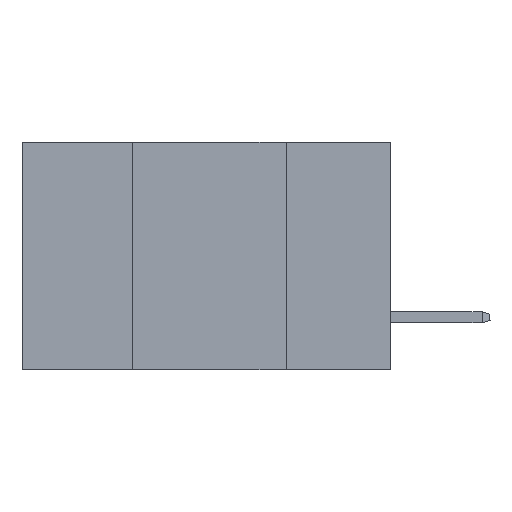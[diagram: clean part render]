
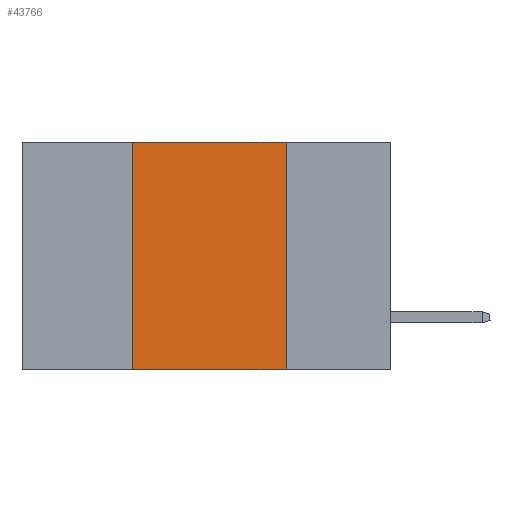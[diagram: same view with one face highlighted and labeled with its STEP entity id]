
A CAD part, left-side view. The second image highlights one B-rep face of the part: STEP entity #43766.
In plain terms, the highlighted planar face has unit normal (-1, 0, 0).
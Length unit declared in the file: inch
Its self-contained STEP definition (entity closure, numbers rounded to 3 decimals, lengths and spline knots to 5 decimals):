
#267 = LINE ( 'NONE', #17194, #22926 ) ;
#1456 = EDGE_CURVE ( 'NONE', #11638, #3674, #27664, .T. ) ;
#1714 = VERTEX_POINT ( 'NONE', #45940 ) ;
#2874 = DIRECTION ( 'NONE',  ( 1., 0., 0. ) ) ;
#2916 = CARTESIAN_POINT ( 'NONE',  ( 0., 0.17, -0.37 ) ) ;
#3674 = VERTEX_POINT ( 'NONE', #2916 ) ;
#4388 = EDGE_CURVE ( 'NONE', #11638, #10976, #28639, .T. ) ;
#6212 = PLANE ( 'NONE',  #17235 ) ;
#9641 = CARTESIAN_POINT ( 'NONE',  ( 0., 0.42, -0.37 ) ) ;
#10976 = VERTEX_POINT ( 'NONE', #39922 ) ;
#11638 = VERTEX_POINT ( 'NONE', #9641 ) ;
#13337 = ORIENTED_EDGE ( 'NONE', *, *, #4388, .F. ) ;
#13346 = EDGE_LOOP ( 'NONE', ( #35513, #32151, #13337, #45210 ) ) ;
#13488 = CARTESIAN_POINT ( 'NONE',  ( 0., 0.17, 0. ) ) ;
#13696 = CARTESIAN_POINT ( 'NONE',  ( 0., 0.42, 0. ) ) ;
#14309 = DIRECTION ( 'NONE',  ( 0., 0., 1. ) ) ;
#16342 = LINE ( 'NONE', #13488, #26004 ) ;
#17088 = CARTESIAN_POINT ( 'NONE',  ( 0., 0.6, 0. ) ) ;
#17194 = CARTESIAN_POINT ( 'NONE',  ( 0., 0.6, 0. ) ) ;
#17235 = AXIS2_PLACEMENT_3D ( 'NONE', #17088, #2874, #39387 ) ;
#17655 = DIRECTION ( 'NONE',  ( 0., -1., 0. ) ) ;
#22926 = VECTOR ( 'NONE', #17655, 39.37008 ) ;
#24451 = DIRECTION ( 'NONE',  ( 0., 0., -1. ) ) ;
#25090 = CARTESIAN_POINT ( 'NONE',  ( 0., 0.6, -0.37 ) ) ;
#26004 = VECTOR ( 'NONE', #24451, 39.37008 ) ;
#27664 = LINE ( 'NONE', #25090, #40850 ) ;
#28623 = DIRECTION ( 'NONE',  ( 0., -1., 0. ) ) ;
#28639 = LINE ( 'NONE', #13696, #37210 ) ;
#32151 = ORIENTED_EDGE ( 'NONE', *, *, #32476, .F. ) ;
#32476 = EDGE_CURVE ( 'NONE', #10976, #1714, #267, .T. ) ;
#35513 = ORIENTED_EDGE ( 'NONE', *, *, #43965, .F. ) ;
#37210 = VECTOR ( 'NONE', #14309, 39.37008 ) ;
#39387 = DIRECTION ( 'NONE',  ( 0., 0., -1. ) ) ;
#39922 = CARTESIAN_POINT ( 'NONE',  ( 0., 0.42, 0. ) ) ;
#40850 = VECTOR ( 'NONE', #28623, 39.37008 ) ;
#42771 = FACE_OUTER_BOUND ( 'NONE', #13346, .T. ) ;
#43766 = ADVANCED_FACE ( 'NONE', ( #42771 ), #6212, .F. ) ;
#43965 = EDGE_CURVE ( 'NONE', #1714, #3674, #16342, .T. ) ;
#45210 = ORIENTED_EDGE ( 'NONE', *, *, #1456, .T. ) ;
#45940 = CARTESIAN_POINT ( 'NONE',  ( 0., 0.17, 0. ) ) ;
